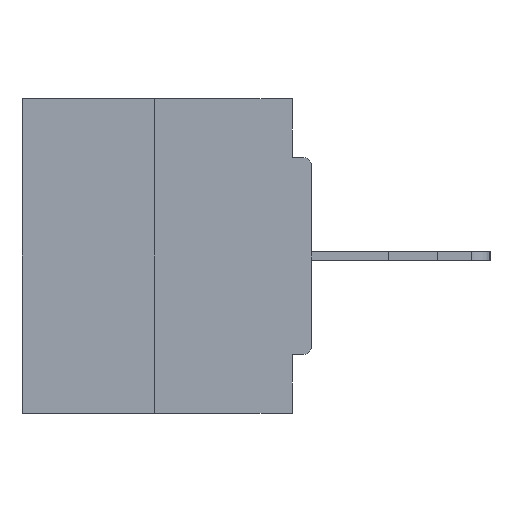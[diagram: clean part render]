
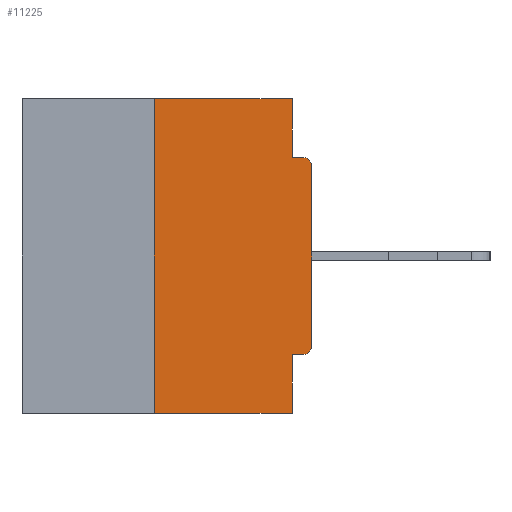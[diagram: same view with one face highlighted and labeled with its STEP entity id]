
A CAD part, left-side view. The second image highlights one B-rep face of the part: STEP entity #11225.
In plain terms, the highlighted planar face has unit normal (-1, 0, 0).
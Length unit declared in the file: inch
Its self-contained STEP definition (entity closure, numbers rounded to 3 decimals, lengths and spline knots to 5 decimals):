
#7 = DIRECTION ( 'NONE',  ( 0., 0., -1. ) ) ;
#555 = DIRECTION ( 'NONE',  ( 0., -1., 0. ) ) ;
#1092 = CARTESIAN_POINT ( 'NONE',  ( 0., 0.25, 0. ) ) ;
#2649 = AXIS2_PLACEMENT_3D ( 'NONE', #31966, #16249, #7 ) ;
#2994 = LINE ( 'NONE', #9461, #19837 ) ;
#3122 = CARTESIAN_POINT ( 'NONE',  ( 0., 0., -0.3915 ) ) ;
#3344 = VECTOR ( 'NONE', #25225, 39.37008 ) ;
#4497 = ORIENTED_EDGE ( 'NONE', *, *, #23903, .T. ) ;
#5334 = DIRECTION ( 'NONE',  ( 0., 0., -1. ) ) ;
#5378 = DIRECTION ( 'NONE',  ( 1., 0., 0. ) ) ;
#5499 = CARTESIAN_POINT ( 'NONE',  ( 0., 0.46, 0. ) ) ;
#5531 = PLANE ( 'NONE',  #8346 ) ;
#5904 = VECTOR ( 'NONE', #30767, 39.37008 ) ;
#6047 = ORIENTED_EDGE ( 'NONE', *, *, #28777, .F. ) ;
#6048 = VERTEX_POINT ( 'NONE', #31547 ) ;
#6401 = CARTESIAN_POINT ( 'NONE',  ( 0., 0.25, -0.5 ) ) ;
#6605 = ORIENTED_EDGE ( 'NONE', *, *, #21295, .F. ) ;
#6739 = LINE ( 'NONE', #17730, #5904 ) ;
#7067 = CARTESIAN_POINT ( 'NONE',  ( 0., 0.031, -0.4065 ) ) ;
#8346 = AXIS2_PLACEMENT_3D ( 'NONE', #5499, #5378, #5334 ) ;
#8465 = CARTESIAN_POINT ( 'NONE',  ( 0., 0.031, -0.5 ) ) ;
#9083 = DIRECTION ( 'NONE',  ( 0., -1., 0. ) ) ;
#9097 = CARTESIAN_POINT ( 'NONE',  ( 0., 0.015, -0.4065 ) ) ;
#9130 = ORIENTED_EDGE ( 'NONE', *, *, #26714, .F. ) ;
#9336 = VERTEX_POINT ( 'NONE', #7067 ) ;
#9461 = CARTESIAN_POINT ( 'NONE',  ( 0., 0.46, -0.5 ) ) ;
#9576 = ORIENTED_EDGE ( 'NONE', *, *, #27713, .T. ) ;
#10030 = CARTESIAN_POINT ( 'NONE',  ( 0., 0.015, -0.3915 ) ) ;
#10057 = VERTEX_POINT ( 'NONE', #25589 ) ;
#10178 = CIRCLE ( 'NONE', #19225, 0.015 ) ;
#10689 = LINE ( 'NONE', #8465, #16889 ) ;
#11225 = ADVANCED_FACE ( 'NONE', ( #33709 ), #5531, .F. ) ;
#11456 = LINE ( 'NONE', #1092, #3344 ) ;
#11892 = VERTEX_POINT ( 'NONE', #3122 ) ;
#11921 = CARTESIAN_POINT ( 'NONE',  ( 0., 0.031, -0.5 ) ) ;
#12225 = VERTEX_POINT ( 'NONE', #9097 ) ;
#12710 = DIRECTION ( 'NONE',  ( 0., 0., -1. ) ) ;
#12790 = VERTEX_POINT ( 'NONE', #13365 ) ;
#13365 = CARTESIAN_POINT ( 'NONE',  ( 0., 0.031, -0.0935 ) ) ;
#14147 = ORIENTED_EDGE ( 'NONE', *, *, #20793, .F. ) ;
#14453 = VERTEX_POINT ( 'NONE', #21913 ) ;
#14482 = EDGE_CURVE ( 'NONE', #12790, #10057, #24961, .T. ) ;
#14859 = VERTEX_POINT ( 'NONE', #20966 ) ;
#14900 = DIRECTION ( 'NONE',  ( 0., -1., 0. ) ) ;
#15831 = CARTESIAN_POINT ( 'NONE',  ( 0., 0.031, 0. ) ) ;
#16249 = DIRECTION ( 'NONE',  ( -1., 0., 0. ) ) ;
#16765 = CARTESIAN_POINT ( 'NONE',  ( 0., 0., -0.0935 ) ) ;
#16798 = VECTOR ( 'NONE', #22640, 39.37008 ) ;
#16889 = VECTOR ( 'NONE', #31975, 39.37008 ) ;
#17416 = CARTESIAN_POINT ( 'NONE',  ( 0., 0., 0. ) ) ;
#17730 = CARTESIAN_POINT ( 'NONE',  ( 0., 0., -0.4065 ) ) ;
#17872 = EDGE_CURVE ( 'NONE', #25717, #19527, #2994, .T. ) ;
#18383 = ORIENTED_EDGE ( 'NONE', *, *, #14482, .F. ) ;
#18438 = VECTOR ( 'NONE', #34161, 39.37008 ) ;
#18959 = EDGE_CURVE ( 'NONE', #25717, #6048, #11456, .T. ) ;
#19225 = AXIS2_PLACEMENT_3D ( 'NONE', #10030, #28476, #12710 ) ;
#19234 = VECTOR ( 'NONE', #9083, 39.37008 ) ;
#19527 = VERTEX_POINT ( 'NONE', #11921 ) ;
#19837 = VECTOR ( 'NONE', #14900, 39.37008 ) ;
#20057 = EDGE_CURVE ( 'NONE', #11892, #14453, #30736, .T. ) ;
#20791 = ORIENTED_EDGE ( 'NONE', *, *, #18959, .F. ) ;
#20793 = EDGE_CURVE ( 'NONE', #12225, #9336, #6739, .T. ) ;
#20966 = CARTESIAN_POINT ( 'NONE',  ( 0., 0.031, 0. ) ) ;
#21295 = EDGE_CURVE ( 'NONE', #6048, #14859, #32305, .T. ) ;
#21913 = CARTESIAN_POINT ( 'NONE',  ( 0., 0., -0.1085 ) ) ;
#22640 = DIRECTION ( 'NONE',  ( 0., 0., 1. ) ) ;
#23903 = EDGE_CURVE ( 'NONE', #14453, #10057, #32301, .T. ) ;
#24227 = EDGE_LOOP ( 'NONE', ( #6605, #20791, #29371, #9130, #14147, #9576, #27750, #4497, #18383, #6047 ) ) ;
#24961 = LINE ( 'NONE', #16765, #25773 ) ;
#25225 = DIRECTION ( 'NONE',  ( 0., 0., 1. ) ) ;
#25371 = LINE ( 'NONE', #15831, #18438 ) ;
#25589 = CARTESIAN_POINT ( 'NONE',  ( 0., 0.015, -0.0935 ) ) ;
#25717 = VERTEX_POINT ( 'NONE', #6401 ) ;
#25773 = VECTOR ( 'NONE', #555, 39.37008 ) ;
#26714 = EDGE_CURVE ( 'NONE', #9336, #19527, #10689, .T. ) ;
#27556 = CARTESIAN_POINT ( 'NONE',  ( 0., 0.46, 0. ) ) ;
#27713 = EDGE_CURVE ( 'NONE', #12225, #11892, #10178, .T. ) ;
#27750 = ORIENTED_EDGE ( 'NONE', *, *, #20057, .T. ) ;
#28476 = DIRECTION ( 'NONE',  ( -1., 0., 0. ) ) ;
#28777 = EDGE_CURVE ( 'NONE', #14859, #12790, #25371, .T. ) ;
#29371 = ORIENTED_EDGE ( 'NONE', *, *, #17872, .T. ) ;
#30736 = LINE ( 'NONE', #17416, #16798 ) ;
#30767 = DIRECTION ( 'NONE',  ( 0., 1., 0. ) ) ;
#31547 = CARTESIAN_POINT ( 'NONE',  ( 0., 0.25, 0. ) ) ;
#31966 = CARTESIAN_POINT ( 'NONE',  ( 0., 0.015, -0.1085 ) ) ;
#31975 = DIRECTION ( 'NONE',  ( 0., 0., -1. ) ) ;
#32301 = CIRCLE ( 'NONE', #2649, 0.015 ) ;
#32305 = LINE ( 'NONE', #27556, #19234 ) ;
#33709 = FACE_OUTER_BOUND ( 'NONE', #24227, .T. ) ;
#34161 = DIRECTION ( 'NONE',  ( 0., 0., -1. ) ) ;
